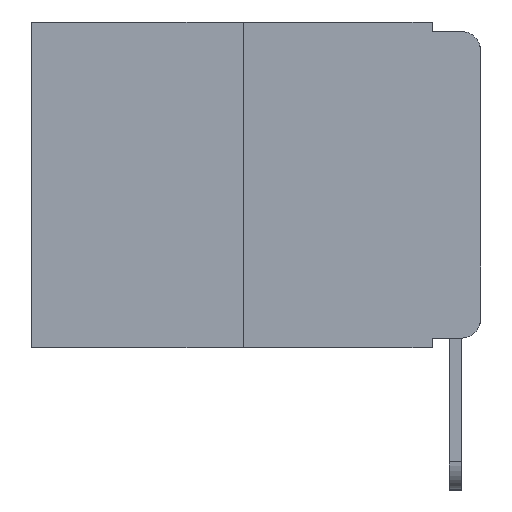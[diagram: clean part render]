
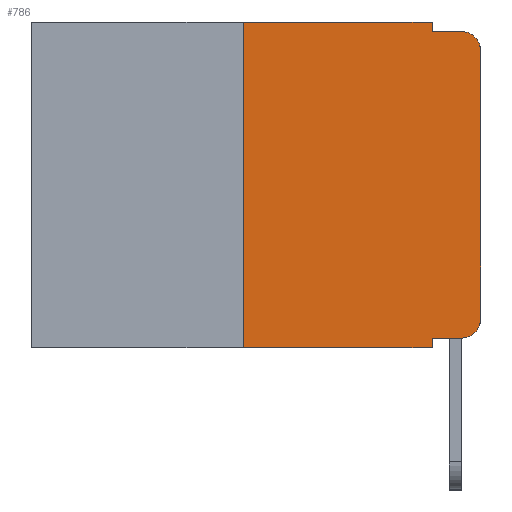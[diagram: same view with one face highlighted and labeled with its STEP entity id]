
A CAD part, left-side view. The second image highlights one B-rep face of the part: STEP entity #786.
In plain terms, the highlighted planar face has unit normal (-1, 0, 0).
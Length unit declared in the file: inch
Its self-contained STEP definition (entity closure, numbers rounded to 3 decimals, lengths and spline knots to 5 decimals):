
#234 = ORIENTED_EDGE ( 'NONE', *, *, #10209, .T. ) ;
#326 = DIRECTION ( 'NONE',  ( 0., 0., -1. ) ) ;
#603 = CIRCLE ( 'NONE', #9756, 0.02 ) ;
#616 = CARTESIAN_POINT ( 'NONE',  ( 0., 0.473, 0. ) ) ;
#637 = VECTOR ( 'NONE', #11225, 39.37008 ) ;
#668 = DIRECTION ( 'NONE',  ( 1., 0., 0. ) ) ;
#786 = ADVANCED_FACE ( 'NONE', ( #2417 ), #4013, .F. ) ;
#920 = ORIENTED_EDGE ( 'NONE', *, *, #12480, .F. ) ;
#1054 = ORIENTED_EDGE ( 'NONE', *, *, #5253, .F. ) ;
#1170 = DIRECTION ( 'NONE',  ( 0., -1., 0. ) ) ;
#1332 = LINE ( 'NONE', #10548, #3989 ) ;
#1650 = LINE ( 'NONE', #11796, #9568 ) ;
#1682 = CARTESIAN_POINT ( 'NONE',  ( 0., 0.051, 0. ) ) ;
#1735 = EDGE_CURVE ( 'NONE', #7078, #11551, #2391, .T. ) ;
#1794 = CARTESIAN_POINT ( 'NONE',  ( 0., 0.25, -0.343 ) ) ;
#1983 = DIRECTION ( 'NONE',  ( 0., -1., 0. ) ) ;
#2284 = VERTEX_POINT ( 'NONE', #5664 ) ;
#2391 = LINE ( 'NONE', #6853, #13234 ) ;
#2417 = FACE_OUTER_BOUND ( 'NONE', #11081, .T. ) ;
#3013 = CARTESIAN_POINT ( 'NONE',  ( 0., 0.02, -0.313 ) ) ;
#3185 = VERTEX_POINT ( 'NONE', #4507 ) ;
#3314 = EDGE_CURVE ( 'NONE', #12005, #10685, #6319, .T. ) ;
#3358 = VERTEX_POINT ( 'NONE', #1794 ) ;
#3387 = VECTOR ( 'NONE', #6487, 39.37008 ) ;
#3831 = EDGE_CURVE ( 'NONE', #3185, #3893, #603, .T. ) ;
#3893 = VERTEX_POINT ( 'NONE', #12607 ) ;
#3987 = LINE ( 'NONE', #4949, #637 ) ;
#3989 = VECTOR ( 'NONE', #11555, 39.37008 ) ;
#3993 = DIRECTION ( 'NONE',  ( -1., 0., 0. ) ) ;
#4013 = PLANE ( 'NONE',  #12665 ) ;
#4114 = EDGE_CURVE ( 'NONE', #7745, #2284, #10541, .T. ) ;
#4163 = DIRECTION ( 'NONE',  ( 0., 0., -1. ) ) ;
#4384 = EDGE_CURVE ( 'NONE', #3893, #12005, #8730, .T. ) ;
#4507 = CARTESIAN_POINT ( 'NONE',  ( 0., 0.02, -0.333 ) ) ;
#4937 = VECTOR ( 'NONE', #326, 39.37008 ) ;
#4949 = CARTESIAN_POINT ( 'NONE',  ( 0., 0.051, -0.01 ) ) ;
#5012 = CARTESIAN_POINT ( 'NONE',  ( 0., 0.051, 0. ) ) ;
#5248 = ORIENTED_EDGE ( 'NONE', *, *, #10729, .F. ) ;
#5253 = EDGE_CURVE ( 'NONE', #8590, #10685, #3987, .T. ) ;
#5535 = VECTOR ( 'NONE', #7236, 39.37008 ) ;
#5664 = CARTESIAN_POINT ( 'NONE',  ( 0., 0.051, -0.343 ) ) ;
#6079 = CARTESIAN_POINT ( 'NONE',  ( 0., 0.051, -0.333 ) ) ;
#6319 = CIRCLE ( 'NONE', #10794, 0.02 ) ;
#6487 = DIRECTION ( 'NONE',  ( 0., 0., 1. ) ) ;
#6853 = CARTESIAN_POINT ( 'NONE',  ( 0., 0.473, 0. ) ) ;
#6947 = ORIENTED_EDGE ( 'NONE', *, *, #4384, .T. ) ;
#7078 = VERTEX_POINT ( 'NONE', #7330 ) ;
#7236 = DIRECTION ( 'NONE',  ( 0., 0., -1. ) ) ;
#7330 = CARTESIAN_POINT ( 'NONE',  ( 0., 0.25, 0. ) ) ;
#7745 = VERTEX_POINT ( 'NONE', #6079 ) ;
#7883 = DIRECTION ( 'NONE',  ( 0., -1., 0. ) ) ;
#7951 = CARTESIAN_POINT ( 'NONE',  ( 0., 0.051, 0. ) ) ;
#8211 = ORIENTED_EDGE ( 'NONE', *, *, #1735, .F. ) ;
#8272 = DIRECTION ( 'NONE',  ( 0., 0., -1. ) ) ;
#8332 = LINE ( 'NONE', #5012, #5535 ) ;
#8487 = CARTESIAN_POINT ( 'NONE',  ( 0., 0.051, -0.333 ) ) ;
#8590 = VERTEX_POINT ( 'NONE', #12526 ) ;
#8730 = LINE ( 'NONE', #12631, #3387 ) ;
#8906 = ORIENTED_EDGE ( 'NONE', *, *, #4114, .F. ) ;
#8994 = LINE ( 'NONE', #8487, #11725 ) ;
#9343 = ORIENTED_EDGE ( 'NONE', *, *, #3314, .T. ) ;
#9568 = VECTOR ( 'NONE', #1170, 39.37008 ) ;
#9691 = ORIENTED_EDGE ( 'NONE', *, *, #13568, .T. ) ;
#9756 = AXIS2_PLACEMENT_3D ( 'NONE', #3013, #10472, #4163 ) ;
#9768 = CARTESIAN_POINT ( 'NONE',  ( 0., 0., -0.03 ) ) ;
#9808 = ORIENTED_EDGE ( 'NONE', *, *, #3831, .T. ) ;
#10209 = EDGE_CURVE ( 'NONE', #7745, #3185, #8994, .T. ) ;
#10295 = CARTESIAN_POINT ( 'NONE',  ( 0., 0.02, -0.01 ) ) ;
#10303 = CARTESIAN_POINT ( 'NONE',  ( 0., 0.02, -0.03 ) ) ;
#10472 = DIRECTION ( 'NONE',  ( -1., 0., 0. ) ) ;
#10541 = LINE ( 'NONE', #7951, #4937 ) ;
#10548 = CARTESIAN_POINT ( 'NONE',  ( 0., 0.25, 0. ) ) ;
#10685 = VERTEX_POINT ( 'NONE', #10295 ) ;
#10729 = EDGE_CURVE ( 'NONE', #11551, #8590, #8332, .T. ) ;
#10794 = AXIS2_PLACEMENT_3D ( 'NONE', #10303, #3993, #11326 ) ;
#11081 = EDGE_LOOP ( 'NONE', ( #6947, #9343, #1054, #5248, #8211, #920, #9691, #8906, #234, #9808 ) ) ;
#11225 = DIRECTION ( 'NONE',  ( 0., -1., 0. ) ) ;
#11326 = DIRECTION ( 'NONE',  ( 0., 0., -1. ) ) ;
#11551 = VERTEX_POINT ( 'NONE', #1682 ) ;
#11555 = DIRECTION ( 'NONE',  ( 0., 0., 1. ) ) ;
#11725 = VECTOR ( 'NONE', #1983, 39.37008 ) ;
#11796 = CARTESIAN_POINT ( 'NONE',  ( 0., 0.473, -0.343 ) ) ;
#12005 = VERTEX_POINT ( 'NONE', #9768 ) ;
#12480 = EDGE_CURVE ( 'NONE', #3358, #7078, #1332, .T. ) ;
#12526 = CARTESIAN_POINT ( 'NONE',  ( 0., 0.051, -0.01 ) ) ;
#12607 = CARTESIAN_POINT ( 'NONE',  ( 0., 0., -0.313 ) ) ;
#12631 = CARTESIAN_POINT ( 'NONE',  ( 0., 0., 0. ) ) ;
#12665 = AXIS2_PLACEMENT_3D ( 'NONE', #616, #668, #8272 ) ;
#13234 = VECTOR ( 'NONE', #7883, 39.37008 ) ;
#13568 = EDGE_CURVE ( 'NONE', #3358, #2284, #1650, .T. ) ;
